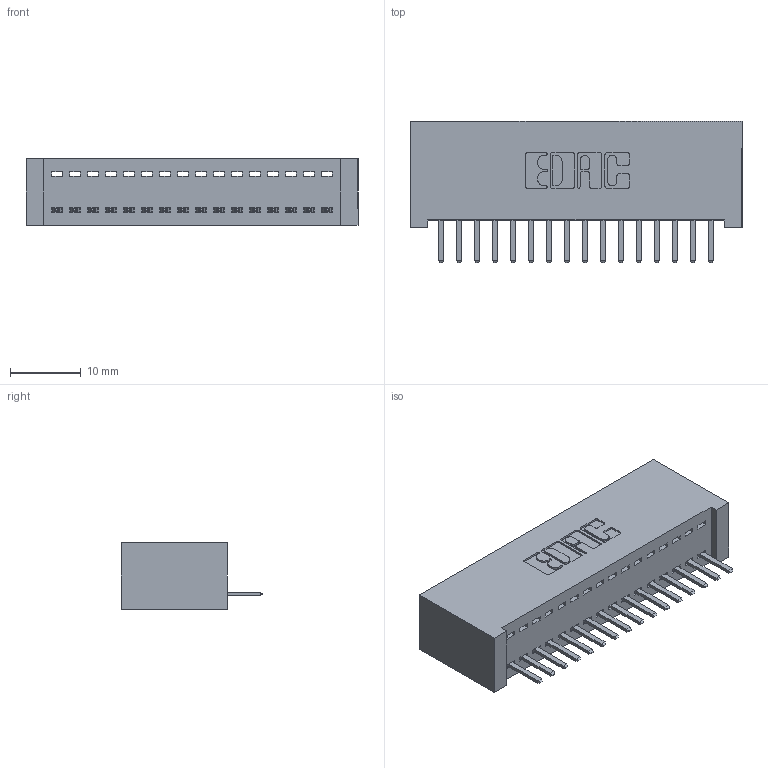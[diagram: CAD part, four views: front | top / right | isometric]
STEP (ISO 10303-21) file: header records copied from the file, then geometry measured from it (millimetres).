
FILE_DESCRIPTION (( 'STEP AP203' ), '1' );
FILE_NAME ('392-016-520-101.STEP', '2019-10-07T02:54:40', ( '' ), ( '' ), 'SwSTEP 2.0', 'SolidWorks 2016', '' );
FILE_SCHEMA (( 'CONFIG_CONTROL_DESIGN' ));
Length unit declared in the file: inch
Products named in the file (3): 392-016-520-101; 342 Part_Lugless; 345-292-001_345-293-120
Assembly tree (17 placements, depth 2):
  392-016-520-101
    342 Part_Lugless
    345-292-001_345-293-120  x16
Bounding box: 46.89 x 20.02 x 9.4 mm (x, y, z)
Volume: 4378.4 mm3; surface area: 6120.1 mm2
Topology: 17 solids, 17 shells, 1094 faces, 3219 edges, 2102 vertices
Faces by surface type: plane 766, cylinder 328
Entity records: 12849 total; most frequent: CARTESIAN_POINT 2238, ORIENTED_EDGE 2178, DIRECTION 1921, EDGE_CURVE 1089, VECTOR 965, LINE 965, VERTEX_POINT 722, AXIS2_PLACEMENT_3D 478
